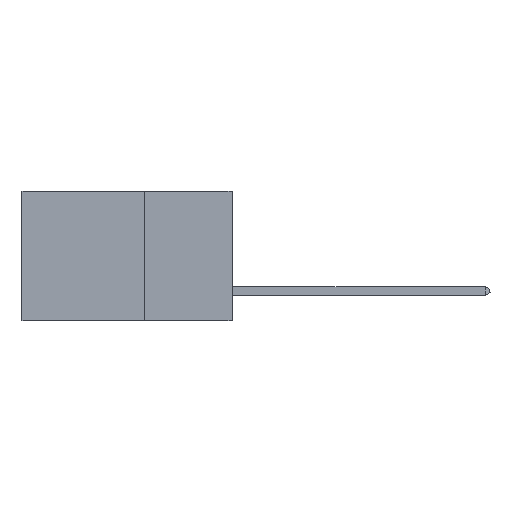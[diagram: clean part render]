
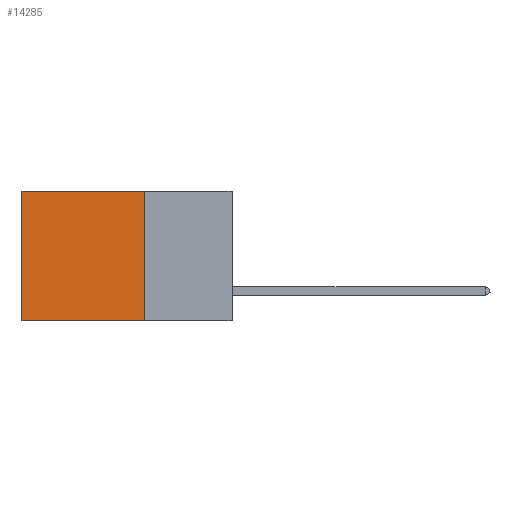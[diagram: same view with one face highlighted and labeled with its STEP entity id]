
A CAD part, left-side view. The second image highlights one B-rep face of the part: STEP entity #14285.
In plain terms, the highlighted planar face has unit normal (-1, 0, 0).
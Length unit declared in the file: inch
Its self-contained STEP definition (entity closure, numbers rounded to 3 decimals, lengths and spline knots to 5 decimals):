
#449 = DIRECTION ( 'NONE',  ( 0., 0., -1. ) ) ;
#581 = EDGE_CURVE ( 'NONE', #2897, #18983, #10837, .T. ) ;
#820 = DIRECTION ( 'NONE',  ( 0., 0., -1. ) ) ;
#1791 = DIRECTION ( 'NONE',  ( 1., 0., 0. ) ) ;
#2536 = ORIENTED_EDGE ( 'NONE', *, *, #6798, .F. ) ;
#2612 = LINE ( 'NONE', #2719, #3082 ) ;
#2719 = CARTESIAN_POINT ( 'NONE',  ( 0.2875, 0.6, 0. ) ) ;
#2801 = AXIS2_PLACEMENT_3D ( 'NONE', #12333, #1791, #449 ) ;
#2897 = VERTEX_POINT ( 'NONE', #4509 ) ;
#2964 = LINE ( 'NONE', #5700, #13792 ) ;
#3082 = VECTOR ( 'NONE', #7417, 39.37008 ) ;
#4509 = CARTESIAN_POINT ( 'NONE',  ( 0.2875, 0.25, 0. ) ) ;
#5700 = CARTESIAN_POINT ( 'NONE',  ( 0.2875, 0.25, 0. ) ) ;
#6710 = DIRECTION ( 'NONE',  ( 0., 1., 0. ) ) ;
#6798 = EDGE_CURVE ( 'NONE', #2897, #18383, #2964, .T. ) ;
#7417 = DIRECTION ( 'NONE',  ( 0., 0., -1. ) ) ;
#8001 = CARTESIAN_POINT ( 'NONE',  ( 0.2875, 0.6, -0.37 ) ) ;
#8938 = CARTESIAN_POINT ( 'NONE',  ( 0.2875, 0.6, 0. ) ) ;
#9901 = DIRECTION ( 'NONE',  ( 0., 1., 0. ) ) ;
#10396 = EDGE_CURVE ( 'NONE', #18983, #19806, #2612, .T. ) ;
#10837 = LINE ( 'NONE', #14871, #12832 ) ;
#11254 = ORIENTED_EDGE ( 'NONE', *, *, #10396, .T. ) ;
#11495 = FACE_OUTER_BOUND ( 'NONE', #13018, .T. ) ;
#12333 = CARTESIAN_POINT ( 'NONE',  ( 0.2875, 0.25, 0. ) ) ;
#12832 = VECTOR ( 'NONE', #9901, 39.37008 ) ;
#13018 = EDGE_LOOP ( 'NONE', ( #11254, #17264, #2536, #17784 ) ) ;
#13546 = PLANE ( 'NONE',  #2801 ) ;
#13792 = VECTOR ( 'NONE', #820, 39.37008 ) ;
#14285 = ADVANCED_FACE ( 'NONE', ( #11495 ), #13546, .F. ) ;
#14497 = CARTESIAN_POINT ( 'NONE',  ( 0.2875, 0.25, -0.37 ) ) ;
#14556 = CARTESIAN_POINT ( 'NONE',  ( 0.2875, 0.25, -0.37 ) ) ;
#14871 = CARTESIAN_POINT ( 'NONE',  ( 0.2875, 0.25, 0. ) ) ;
#15259 = VECTOR ( 'NONE', #6710, 39.37008 ) ;
#17264 = ORIENTED_EDGE ( 'NONE', *, *, #17938, .F. ) ;
#17784 = ORIENTED_EDGE ( 'NONE', *, *, #581, .T. ) ;
#17938 = EDGE_CURVE ( 'NONE', #18383, #19806, #19395, .T. ) ;
#18383 = VERTEX_POINT ( 'NONE', #14497 ) ;
#18983 = VERTEX_POINT ( 'NONE', #8938 ) ;
#19395 = LINE ( 'NONE', #14556, #15259 ) ;
#19806 = VERTEX_POINT ( 'NONE', #8001 ) ;
